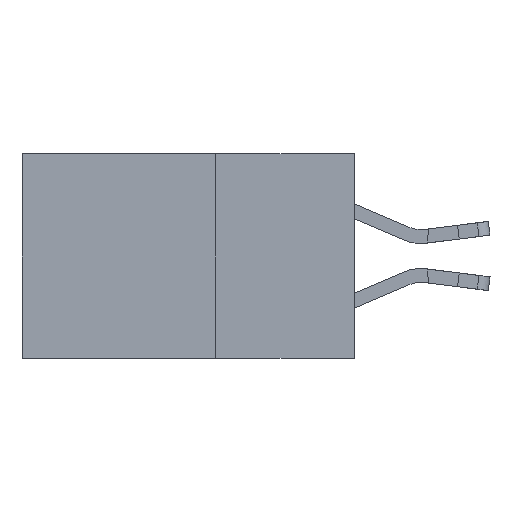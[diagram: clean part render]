
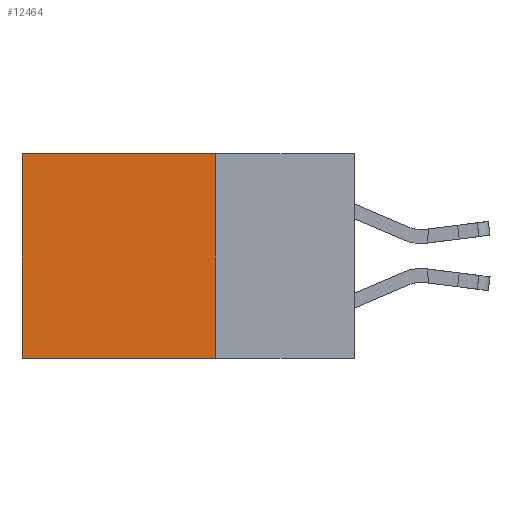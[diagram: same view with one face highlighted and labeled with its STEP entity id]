
A CAD part, left-side view. The second image highlights one B-rep face of the part: STEP entity #12464.
In plain terms, the highlighted planar face has unit normal (-1, 0, 0).
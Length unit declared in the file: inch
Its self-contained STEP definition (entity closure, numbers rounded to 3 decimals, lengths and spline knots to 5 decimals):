
#134 = DIRECTION ( 'NONE',  ( 0., 0., -1. ) ) ;
#413 = ORIENTED_EDGE ( 'NONE', *, *, #12641, .T. ) ;
#508 = LINE ( 'NONE', #9039, #7795 ) ;
#637 = AXIS2_PLACEMENT_3D ( 'NONE', #2738, #12746, #4173 ) ;
#1827 = DIRECTION ( 'NONE',  ( 0., 1., 0. ) ) ;
#2278 = ORIENTED_EDGE ( 'NONE', *, *, #17777, .F. ) ;
#2738 = CARTESIAN_POINT ( 'NONE',  ( 0.2615, 0.25, -0.37 ) ) ;
#3059 = CARTESIAN_POINT ( 'NONE',  ( 0.2615, 0.6, -0.37 ) ) ;
#4173 = DIRECTION ( 'NONE',  ( 0., 0., -1. ) ) ;
#4598 = LINE ( 'NONE', #10139, #8003 ) ;
#5774 = DIRECTION ( 'NONE',  ( 0., 0., -1. ) ) ;
#6177 = VERTEX_POINT ( 'NONE', #11784 ) ;
#6192 = VECTOR ( 'NONE', #13665, 39.37008 ) ;
#6306 = FACE_OUTER_BOUND ( 'NONE', #15459, .T. ) ;
#6929 = ORIENTED_EDGE ( 'NONE', *, *, #18140, .F. ) ;
#6952 = VECTOR ( 'NONE', #134, 39.37008 ) ;
#7416 = LINE ( 'NONE', #3059, #6952 ) ;
#7555 = CARTESIAN_POINT ( 'NONE',  ( 0.2615, 0.25, 0. ) ) ;
#7655 = VERTEX_POINT ( 'NONE', #7555 ) ;
#7795 = VECTOR ( 'NONE', #1827, 39.37008 ) ;
#8003 = VECTOR ( 'NONE', #5774, 39.37008 ) ;
#8371 = CARTESIAN_POINT ( 'NONE',  ( 0.2615, 0.25, -0.37 ) ) ;
#9039 = CARTESIAN_POINT ( 'NONE',  ( 0.2615, 0.25, 0. ) ) ;
#10139 = CARTESIAN_POINT ( 'NONE',  ( 0.2615, 0.25, -0.37 ) ) ;
#10245 = ORIENTED_EDGE ( 'NONE', *, *, #14702, .T. ) ;
#10933 = VERTEX_POINT ( 'NONE', #8371 ) ;
#11623 = VERTEX_POINT ( 'NONE', #16833 ) ;
#11784 = CARTESIAN_POINT ( 'NONE',  ( 0.2615, 0.6, -0.37 ) ) ;
#12213 = CARTESIAN_POINT ( 'NONE',  ( 0.2615, 0.25, -0.37 ) ) ;
#12464 = ADVANCED_FACE ( 'NONE', ( #6306 ), #18451, .F. ) ;
#12641 = EDGE_CURVE ( 'NONE', #11623, #6177, #7416, .T. ) ;
#12746 = DIRECTION ( 'NONE',  ( 1., 0., 0. ) ) ;
#13665 = DIRECTION ( 'NONE',  ( 0., 1., 0. ) ) ;
#14702 = EDGE_CURVE ( 'NONE', #7655, #11623, #508, .T. ) ;
#15459 = EDGE_LOOP ( 'NONE', ( #413, #6929, #2278, #10245 ) ) ;
#16833 = CARTESIAN_POINT ( 'NONE',  ( 0.2615, 0.6, 0. ) ) ;
#17614 = LINE ( 'NONE', #12213, #6192 ) ;
#17777 = EDGE_CURVE ( 'NONE', #7655, #10933, #4598, .T. ) ;
#18140 = EDGE_CURVE ( 'NONE', #10933, #6177, #17614, .T. ) ;
#18451 = PLANE ( 'NONE',  #637 ) ;
